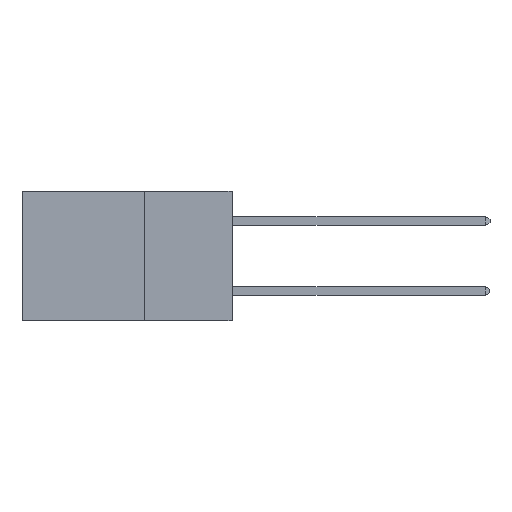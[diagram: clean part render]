
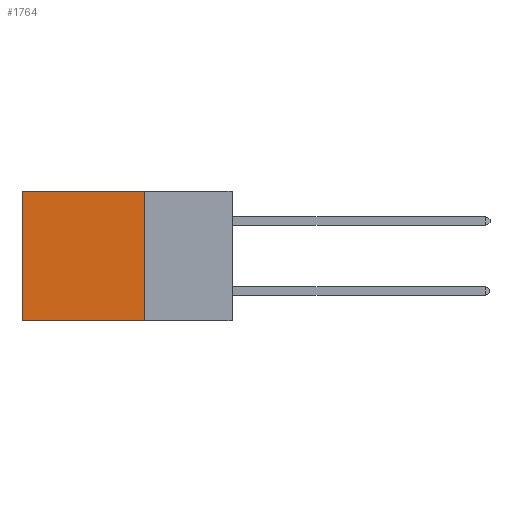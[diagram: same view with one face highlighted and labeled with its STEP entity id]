
A CAD part, left-side view. The second image highlights one B-rep face of the part: STEP entity #1764.
In plain terms, the highlighted planar face has unit normal (-1, 0, 0).
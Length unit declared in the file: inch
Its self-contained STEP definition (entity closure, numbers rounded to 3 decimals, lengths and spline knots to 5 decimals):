
#213 = CARTESIAN_POINT ( 'NONE',  ( 0.2875, 0.6, 0. ) ) ;
#222 = FACE_OUTER_BOUND ( 'NONE', #18878, .T. ) ;
#1050 = CARTESIAN_POINT ( 'NONE',  ( 0.2875, 0.25, -0.37 ) ) ;
#1764 = ADVANCED_FACE ( 'NONE', ( #222 ), #2801, .F. ) ;
#2414 = DIRECTION ( 'NONE',  ( 0., 0., -1. ) ) ;
#2801 = PLANE ( 'NONE',  #4878 ) ;
#3208 = VECTOR ( 'NONE', #2414, 39.37008 ) ;
#3259 = CARTESIAN_POINT ( 'NONE',  ( 0.2875, 0.6, 0. ) ) ;
#3648 = VERTEX_POINT ( 'NONE', #1050 ) ;
#4370 = ORIENTED_EDGE ( 'NONE', *, *, #15399, .F. ) ;
#4788 = VECTOR ( 'NONE', #11855, 39.37008 ) ;
#4878 = AXIS2_PLACEMENT_3D ( 'NONE', #6124, #9442, #20749 ) ;
#6124 = CARTESIAN_POINT ( 'NONE',  ( 0.2875, 0.25, 0. ) ) ;
#6317 = VERTEX_POINT ( 'NONE', #3259 ) ;
#6321 = EDGE_CURVE ( 'NONE', #6550, #6317, #15193, .T. ) ;
#6550 = VERTEX_POINT ( 'NONE', #8860 ) ;
#6578 = CARTESIAN_POINT ( 'NONE',  ( 0.2875, 0.25, 0. ) ) ;
#8020 = ORIENTED_EDGE ( 'NONE', *, *, #9622, .T. ) ;
#8115 = LINE ( 'NONE', #10666, #3208 ) ;
#8243 = DIRECTION ( 'NONE',  ( 0., 1., 0. ) ) ;
#8377 = CARTESIAN_POINT ( 'NONE',  ( 0.2875, 0.25, -0.37 ) ) ;
#8860 = CARTESIAN_POINT ( 'NONE',  ( 0.2875, 0.25, 0. ) ) ;
#9442 = DIRECTION ( 'NONE',  ( 1., 0., 0. ) ) ;
#9622 = EDGE_CURVE ( 'NONE', #6317, #12793, #17782, .T. ) ;
#10051 = DIRECTION ( 'NONE',  ( 0., 1., 0. ) ) ;
#10126 = EDGE_CURVE ( 'NONE', #6550, #3648, #8115, .T. ) ;
#10666 = CARTESIAN_POINT ( 'NONE',  ( 0.2875, 0.25, 0. ) ) ;
#10893 = VECTOR ( 'NONE', #8243, 39.37008 ) ;
#11075 = CARTESIAN_POINT ( 'NONE',  ( 0.2875, 0.6, -0.37 ) ) ;
#11855 = DIRECTION ( 'NONE',  ( 0., 0., -1. ) ) ;
#12793 = VERTEX_POINT ( 'NONE', #11075 ) ;
#14689 = LINE ( 'NONE', #8377, #17938 ) ;
#15193 = LINE ( 'NONE', #6578, #10893 ) ;
#15399 = EDGE_CURVE ( 'NONE', #3648, #12793, #14689, .T. ) ;
#16138 = ORIENTED_EDGE ( 'NONE', *, *, #10126, .F. ) ;
#17782 = LINE ( 'NONE', #213, #4788 ) ;
#17938 = VECTOR ( 'NONE', #10051, 39.37008 ) ;
#18878 = EDGE_LOOP ( 'NONE', ( #8020, #4370, #16138, #19015 ) ) ;
#19015 = ORIENTED_EDGE ( 'NONE', *, *, #6321, .T. ) ;
#20749 = DIRECTION ( 'NONE',  ( 0., 0., -1. ) ) ;
